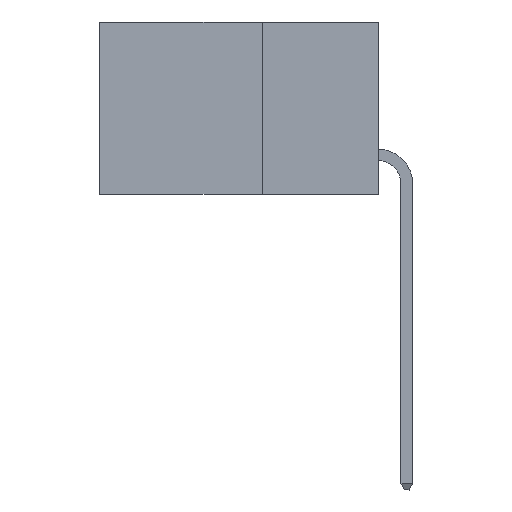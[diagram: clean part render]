
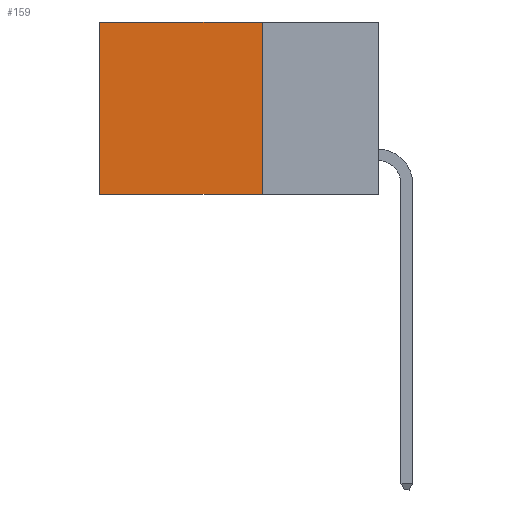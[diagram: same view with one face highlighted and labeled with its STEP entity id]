
A CAD part, left-side view. The second image highlights one B-rep face of the part: STEP entity #159.
In plain terms, the highlighted planar face has unit normal (-1, 0, 0).
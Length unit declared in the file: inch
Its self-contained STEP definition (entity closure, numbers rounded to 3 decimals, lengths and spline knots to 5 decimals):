
#159 = ADVANCED_FACE ( 'NONE', ( #6689 ), #10899, .F. ) ;
#404 = DIRECTION ( 'NONE',  ( 0., 1., 0. ) ) ;
#914 = CARTESIAN_POINT ( 'NONE',  ( 0.298, 0.6, 0. ) ) ;
#1513 = DIRECTION ( 'NONE',  ( 0., 0., -1. ) ) ;
#1534 = DIRECTION ( 'NONE',  ( 0., 0., -1. ) ) ;
#1991 = CARTESIAN_POINT ( 'NONE',  ( 0.298, 0.6, 0. ) ) ;
#2120 = DIRECTION ( 'NONE',  ( 0., 0., -1. ) ) ;
#2434 = VECTOR ( 'NONE', #1513, 39.37008 ) ;
#2867 = AXIS2_PLACEMENT_3D ( 'NONE', #12934, #12981, #1534 ) ;
#2975 = CARTESIAN_POINT ( 'NONE',  ( 0.298, 0.25, 0. ) ) ;
#2998 = LINE ( 'NONE', #3433, #10999 ) ;
#3091 = LINE ( 'NONE', #5640, #2434 ) ;
#3356 = EDGE_CURVE ( 'NONE', #5718, #10595, #2998, .T. ) ;
#3433 = CARTESIAN_POINT ( 'NONE',  ( 0.298, 0.25, -0.37 ) ) ;
#3469 = ORIENTED_EDGE ( 'NONE', *, *, #3356, .F. ) ;
#3819 = ORIENTED_EDGE ( 'NONE', *, *, #7786, .T. ) ;
#3962 = DIRECTION ( 'NONE',  ( 0., 1., 0. ) ) ;
#4033 = VECTOR ( 'NONE', #3962, 39.37008 ) ;
#4986 = EDGE_CURVE ( 'NONE', #12557, #8088, #6815, .T. ) ;
#5640 = CARTESIAN_POINT ( 'NONE',  ( 0.298, 0.25, 0. ) ) ;
#5718 = VERTEX_POINT ( 'NONE', #6392 ) ;
#5734 = LINE ( 'NONE', #1991, #5888 ) ;
#5888 = VECTOR ( 'NONE', #2120, 39.37008 ) ;
#6113 = EDGE_LOOP ( 'NONE', ( #3819, #3469, #7701, #6842 ) ) ;
#6392 = CARTESIAN_POINT ( 'NONE',  ( 0.298, 0.25, -0.37 ) ) ;
#6689 = FACE_OUTER_BOUND ( 'NONE', #6113, .T. ) ;
#6759 = CARTESIAN_POINT ( 'NONE',  ( 0.298, 0.6, -0.37 ) ) ;
#6815 = LINE ( 'NONE', #8239, #4033 ) ;
#6842 = ORIENTED_EDGE ( 'NONE', *, *, #4986, .T. ) ;
#7701 = ORIENTED_EDGE ( 'NONE', *, *, #9149, .F. ) ;
#7786 = EDGE_CURVE ( 'NONE', #8088, #10595, #5734, .T. ) ;
#8088 = VERTEX_POINT ( 'NONE', #914 ) ;
#8239 = CARTESIAN_POINT ( 'NONE',  ( 0.298, 0.25, 0. ) ) ;
#9149 = EDGE_CURVE ( 'NONE', #12557, #5718, #3091, .T. ) ;
#10595 = VERTEX_POINT ( 'NONE', #6759 ) ;
#10899 = PLANE ( 'NONE',  #2867 ) ;
#10999 = VECTOR ( 'NONE', #404, 39.37008 ) ;
#12557 = VERTEX_POINT ( 'NONE', #2975 ) ;
#12934 = CARTESIAN_POINT ( 'NONE',  ( 0.298, 0.25, 0. ) ) ;
#12981 = DIRECTION ( 'NONE',  ( 1., 0., 0. ) ) ;
